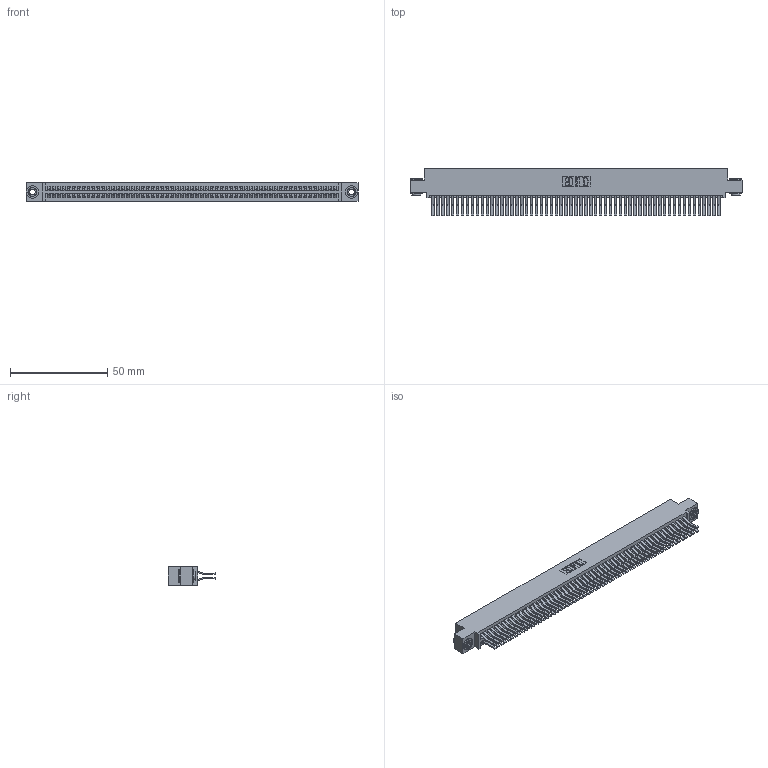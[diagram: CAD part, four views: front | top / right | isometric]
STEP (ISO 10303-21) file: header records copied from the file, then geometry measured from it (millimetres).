
FILE_DESCRIPTION (( 'STEP AP203' ), '1' );
FILE_NAME ('845-118-560-503.STEP', '2018-11-21T00:08:52', ( '' ), ( '' ), 'SwSTEP 2.0', 'SolidWorks 2016', '' );
FILE_SCHEMA (( 'CONFIG_CONTROL_DESIGN' ));
Length unit declared in the file: inch
Products named in the file (4): 845 Part_0.110 Offset - 0.156 Dia-TH; 345-292-001_560 Tail; 345-250-002_345-250-002-102; 845-118-560-503
Assembly tree (121 placements, depth 2):
  845-118-560-503
    845 Part_0.110 Offset - 0.156 Dia-TH
    345-292-001_560 Tail  x118
    345-250-002_345-250-002-102  x2
Bounding box: 171.07 x 24.45 x 9.4 mm (x, y, z)
Volume: 17495.1 mm3; surface area: 28476.9 mm2
Topology: 121 solids, 121 shells, 6304 faces, 18719 edges, 12318 vertices
Faces by surface type: plane 3988, cylinder 2308, cone 8
Entity records: 44874 total; most frequent: CARTESIAN_POINT 7483, ORIENTED_EDGE 7410, DIRECTION 6611, EDGE_CURVE 3705, VECTOR 3309, LINE 3309, VERTEX_POINT 2466, AXIS2_PLACEMENT_3D 1651
